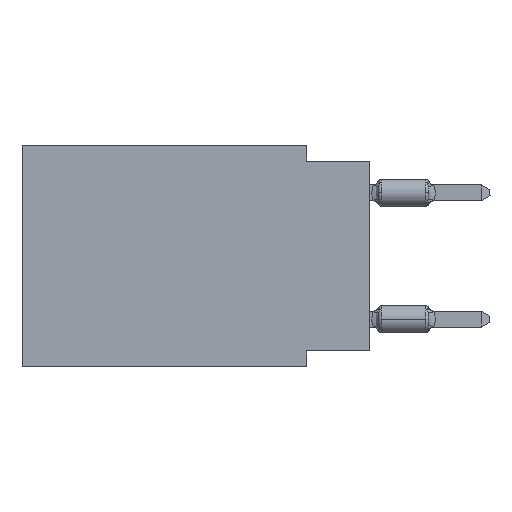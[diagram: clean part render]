
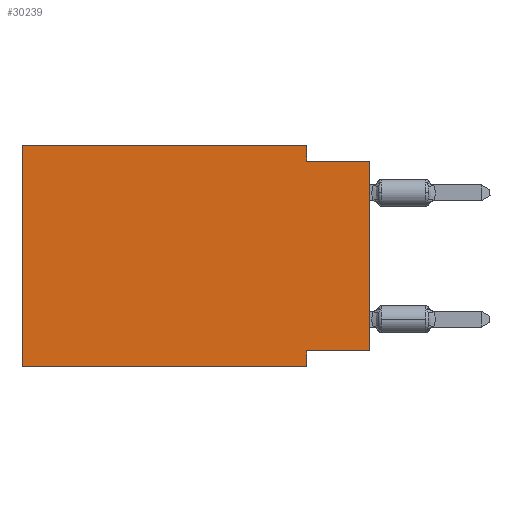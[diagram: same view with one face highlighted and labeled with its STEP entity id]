
A CAD part, left-side view. The second image highlights one B-rep face of the part: STEP entity #30239.
In plain terms, the highlighted planar face has unit normal (-1, 0, 0).
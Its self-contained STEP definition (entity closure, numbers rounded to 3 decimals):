
#1942 = EDGE_LOOP ( 'NONE', ( #44237, #54723, #17585, #51435, #43202, #40651, #45879, #3988 ) ) ;
#2539 = LINE ( 'NONE', #44812, #33288 ) ;
#2589 = DIRECTION ( 'NONE',  ( 0., 0., -1. ) ) ;
#2887 = CARTESIAN_POINT ( 'NONE',  ( 0., 0., -0.635 ) ) ;
#3988 = ORIENTED_EDGE ( 'NONE', *, *, #35607, .F. ) ;
#4343 = LINE ( 'NONE', #2887, #47718 ) ;
#4632 = LINE ( 'NONE', #5244, #34097 ) ;
#4955 = CARTESIAN_POINT ( 'NONE',  ( 0., 2.54, -8.89 ) ) ;
#5244 = CARTESIAN_POINT ( 'NONE',  ( 0., 0., -8.255 ) ) ;
#9651 = VECTOR ( 'NONE', #59468, 1000. ) ;
#10787 = EDGE_CURVE ( 'NONE', #34125, #21991, #45192, .T. ) ;
#15327 = EDGE_CURVE ( 'NONE', #27602, #31320, #4343, .T. ) ;
#16762 = EDGE_CURVE ( 'NONE', #50228, #21991, #54179, .T. ) ;
#17585 = ORIENTED_EDGE ( 'NONE', *, *, #23545, .F. ) ;
#18553 = DIRECTION ( 'NONE',  ( 0., 0., -1. ) ) ;
#18621 = DIRECTION ( 'NONE',  ( 1., 0., 0. ) ) ;
#21193 = DIRECTION ( 'NONE',  ( 0., 0., 1. ) ) ;
#21991 = VERTEX_POINT ( 'NONE', #4955 ) ;
#23248 = VERTEX_POINT ( 'NONE', #28889 ) ;
#23284 = FACE_OUTER_BOUND ( 'NONE', #1942, .T. ) ;
#23521 = LINE ( 'NONE', #28502, #24274 ) ;
#23545 = EDGE_CURVE ( 'NONE', #49811, #27602, #23521, .T. ) ;
#24274 = VECTOR ( 'NONE', #18553, 1000. ) ;
#27171 = DIRECTION ( 'NONE',  ( 0., -1., 0. ) ) ;
#27602 = VERTEX_POINT ( 'NONE', #47705 ) ;
#27635 = DIRECTION ( 'NONE',  ( 0., -1., 0. ) ) ;
#28502 = CARTESIAN_POINT ( 'NONE',  ( 0., 2.54, 0. ) ) ;
#28889 = CARTESIAN_POINT ( 'NONE',  ( 0., 13.97, 0. ) ) ;
#29089 = EDGE_CURVE ( 'NONE', #34125, #23248, #34150, .T. ) ;
#30143 = AXIS2_PLACEMENT_3D ( 'NONE', #51238, #18621, #55597 ) ;
#30239 = ADVANCED_FACE ( 'NONE', ( #23284 ), #32308, .F. ) ;
#30576 = CARTESIAN_POINT ( 'NONE',  ( 0., 13.97, -8.89 ) ) ;
#31320 = VERTEX_POINT ( 'NONE', #34640 ) ;
#31508 = CARTESIAN_POINT ( 'NONE',  ( 0., 13.97, -8.89 ) ) ;
#32308 = PLANE ( 'NONE',  #30143 ) ;
#32312 = EDGE_CURVE ( 'NONE', #23248, #49811, #53623, .T. ) ;
#33288 = VECTOR ( 'NONE', #21193, 1000. ) ;
#34097 = VECTOR ( 'NONE', #41905, 1000. ) ;
#34125 = VERTEX_POINT ( 'NONE', #30576 ) ;
#34150 = LINE ( 'NONE', #57441, #59767 ) ;
#34191 = CARTESIAN_POINT ( 'NONE',  ( 0., 2.54, 0. ) ) ;
#34640 = CARTESIAN_POINT ( 'NONE',  ( 0., 0., -0.635 ) ) ;
#35234 = CARTESIAN_POINT ( 'NONE',  ( 0., 2.54, -8.89 ) ) ;
#35607 = EDGE_CURVE ( 'NONE', #39044, #50228, #4632, .T. ) ;
#39044 = VERTEX_POINT ( 'NONE', #57689 ) ;
#40651 = ORIENTED_EDGE ( 'NONE', *, *, #10787, .T. ) ;
#41905 = DIRECTION ( 'NONE',  ( 0., 1., 0. ) ) ;
#43202 = ORIENTED_EDGE ( 'NONE', *, *, #29089, .F. ) ;
#44237 = ORIENTED_EDGE ( 'NONE', *, *, #59329, .T. ) ;
#44812 = CARTESIAN_POINT ( 'NONE',  ( 0., 0., 0. ) ) ;
#45192 = LINE ( 'NONE', #31508, #9651 ) ;
#45879 = ORIENTED_EDGE ( 'NONE', *, *, #16762, .F. ) ;
#47157 = CARTESIAN_POINT ( 'NONE',  ( 0., 2.54, -8.255 ) ) ;
#47705 = CARTESIAN_POINT ( 'NONE',  ( 0., 2.54, -0.635 ) ) ;
#47718 = VECTOR ( 'NONE', #27635, 1000. ) ;
#49717 = VECTOR ( 'NONE', #27171, 1000. ) ;
#49811 = VERTEX_POINT ( 'NONE', #34191 ) ;
#50228 = VERTEX_POINT ( 'NONE', #47157 ) ;
#51238 = CARTESIAN_POINT ( 'NONE',  ( 0., 13.97, 0. ) ) ;
#51435 = ORIENTED_EDGE ( 'NONE', *, *, #32312, .F. ) ;
#52776 = DIRECTION ( 'NONE',  ( 0., 0., 1. ) ) ;
#53623 = LINE ( 'NONE', #55429, #49717 ) ;
#54179 = LINE ( 'NONE', #35234, #57344 ) ;
#54723 = ORIENTED_EDGE ( 'NONE', *, *, #15327, .F. ) ;
#55429 = CARTESIAN_POINT ( 'NONE',  ( 0., 13.97, 0. ) ) ;
#55597 = DIRECTION ( 'NONE',  ( 0., 0., -1. ) ) ;
#57344 = VECTOR ( 'NONE', #2589, 1000. ) ;
#57441 = CARTESIAN_POINT ( 'NONE',  ( 0., 13.97, 0. ) ) ;
#57689 = CARTESIAN_POINT ( 'NONE',  ( 0., 0., -8.255 ) ) ;
#59329 = EDGE_CURVE ( 'NONE', #39044, #31320, #2539, .T. ) ;
#59468 = DIRECTION ( 'NONE',  ( 0., -1., 0. ) ) ;
#59767 = VECTOR ( 'NONE', #52776, 1000. ) ;
